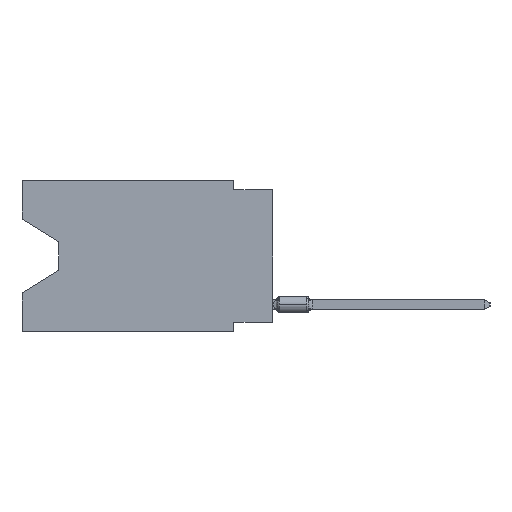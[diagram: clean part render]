
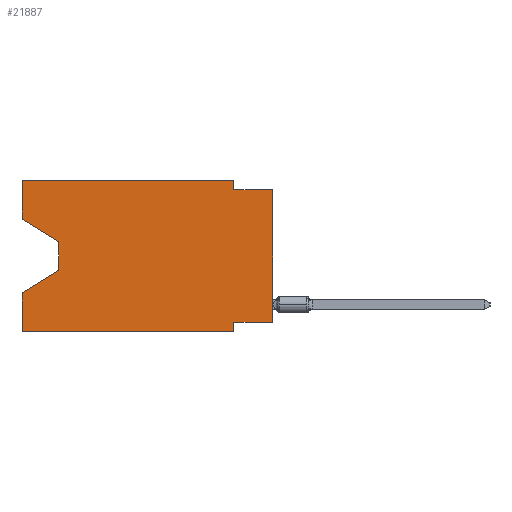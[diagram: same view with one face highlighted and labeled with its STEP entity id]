
A CAD part, left-side view. The second image highlights one B-rep face of the part: STEP entity #21887.
In plain terms, the highlighted planar face has unit normal (-1, 0, 0).
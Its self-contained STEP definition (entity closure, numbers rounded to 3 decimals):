
#831 = VERTEX_POINT ( 'NONE', #34615 ) ;
#1545 = LINE ( 'NONE', #26034, #27329 ) ;
#1785 = CARTESIAN_POINT ( 'NONE',  ( 0., 16.383, -9.906 ) ) ;
#2876 = AXIS2_PLACEMENT_3D ( 'NONE', #51120, #46877, #22471 ) ;
#3183 = LINE ( 'NONE', #36158, #4420 ) ;
#3399 = ORIENTED_EDGE ( 'NONE', *, *, #40823, .T. ) ;
#4256 = ORIENTED_EDGE ( 'NONE', *, *, #48733, .F. ) ;
#4420 = VECTOR ( 'NONE', #36419, 1000. ) ;
#5033 = VERTEX_POINT ( 'NONE', #38835 ) ;
#5280 = CARTESIAN_POINT ( 'NONE',  ( 0., 0., 0. ) ) ;
#5468 = CARTESIAN_POINT ( 'NONE',  ( 0., 0., -9.271 ) ) ;
#7400 = VECTOR ( 'NONE', #24288, 1000. ) ;
#10766 = EDGE_CURVE ( 'NONE', #42158, #831, #1545, .T. ) ;
#10770 = FACE_OUTER_BOUND ( 'NONE', #13644, .T. ) ;
#11017 = ORIENTED_EDGE ( 'NONE', *, *, #44623, .F. ) ;
#11124 = VERTEX_POINT ( 'NONE', #34061 ) ;
#12025 = ORIENTED_EDGE ( 'NONE', *, *, #39941, .T. ) ;
#12533 = CARTESIAN_POINT ( 'NONE',  ( 0., 13.97, -4.013 ) ) ;
#12757 = VERTEX_POINT ( 'NONE', #39662 ) ;
#12951 = VECTOR ( 'NONE', #42785, 1000. ) ;
#13255 = LINE ( 'NONE', #5280, #24822 ) ;
#13481 = ORIENTED_EDGE ( 'NONE', *, *, #10766, .F. ) ;
#13644 = EDGE_LOOP ( 'NONE', ( #12025, #32286, #3399, #4256, #22071, #27933, #26501, #36245, #28026, #23104, #11017, #13481 ) ) ;
#13755 = DIRECTION ( 'NONE',  ( 0., 0., -1. ) ) ;
#15099 = DIRECTION ( 'NONE',  ( 0., 0., 1. ) ) ;
#16007 = VERTEX_POINT ( 'NONE', #45386 ) ;
#16829 = LINE ( 'NONE', #44961, #7400 ) ;
#17113 = VECTOR ( 'NONE', #44923, 1000. ) ;
#17151 = VERTEX_POINT ( 'NONE', #1785 ) ;
#17967 = DIRECTION ( 'NONE',  ( 0., -1., 0. ) ) ;
#19149 = CARTESIAN_POINT ( 'NONE',  ( 0., 2.54, -9.906 ) ) ;
#20970 = VECTOR ( 'NONE', #17967, 1000. ) ;
#21887 = ADVANCED_FACE ( 'NONE', ( #10770 ), #26980, .F. ) ;
#22071 = ORIENTED_EDGE ( 'NONE', *, *, #27393, .T. ) ;
#22471 = DIRECTION ( 'NONE',  ( 0., 0., -1. ) ) ;
#23104 = ORIENTED_EDGE ( 'NONE', *, *, #23711, .F. ) ;
#23711 = EDGE_CURVE ( 'NONE', #16007, #33306, #38208, .T. ) ;
#23868 = LINE ( 'NONE', #39273, #49271 ) ;
#24238 = DIRECTION ( 'NONE',  ( 0., 0.855, -0.519 ) ) ;
#24288 = DIRECTION ( 'NONE',  ( 0., -0.855, -0.519 ) ) ;
#24591 = VECTOR ( 'NONE', #24238, 1000. ) ;
#24822 = VECTOR ( 'NONE', #33198, 1000. ) ;
#25986 = CARTESIAN_POINT ( 'NONE',  ( 0., 16.383, 0. ) ) ;
#26034 = CARTESIAN_POINT ( 'NONE',  ( 0., 16.383, 0. ) ) ;
#26501 = ORIENTED_EDGE ( 'NONE', *, *, #43029, .F. ) ;
#26977 = CARTESIAN_POINT ( 'NONE',  ( 0., 0., -9.271 ) ) ;
#26980 = PLANE ( 'NONE',  #2876 ) ;
#27329 = VECTOR ( 'NONE', #30273, 1000. ) ;
#27393 = EDGE_CURVE ( 'NONE', #17151, #41186, #3183, .T. ) ;
#27529 = EDGE_CURVE ( 'NONE', #36284, #5033, #13255, .T. ) ;
#27933 = ORIENTED_EDGE ( 'NONE', *, *, #32968, .F. ) ;
#27949 = LINE ( 'NONE', #32206, #24591 ) ;
#28026 = ORIENTED_EDGE ( 'NONE', *, *, #46374, .F. ) ;
#28791 = CARTESIAN_POINT ( 'NONE',  ( 0., 16.383, -2.546 ) ) ;
#29689 = DIRECTION ( 'NONE',  ( 0., -1., 0. ) ) ;
#30273 = DIRECTION ( 'NONE',  ( 0., 0., 1. ) ) ;
#31568 = EDGE_CURVE ( 'NONE', #43989, #12757, #32733, .T. ) ;
#31872 = CARTESIAN_POINT ( 'NONE',  ( 0., 13.97, -4.013 ) ) ;
#32206 = CARTESIAN_POINT ( 'NONE',  ( 0., 13.97, -5.893 ) ) ;
#32286 = ORIENTED_EDGE ( 'NONE', *, *, #31568, .T. ) ;
#32733 = LINE ( 'NONE', #12533, #17113 ) ;
#32968 = EDGE_CURVE ( 'NONE', #11124, #41186, #42269, .T. ) ;
#33198 = DIRECTION ( 'NONE',  ( 0., 0., 1. ) ) ;
#33306 = VERTEX_POINT ( 'NONE', #40872 ) ;
#33954 = LINE ( 'NONE', #25986, #50386 ) ;
#34061 = CARTESIAN_POINT ( 'NONE',  ( 0., 2.54, -9.271 ) ) ;
#34615 = CARTESIAN_POINT ( 'NONE',  ( 0., 16.383, 0. ) ) ;
#36158 = CARTESIAN_POINT ( 'NONE',  ( 0., 16.383, -9.906 ) ) ;
#36245 = ORIENTED_EDGE ( 'NONE', *, *, #27529, .T. ) ;
#36284 = VERTEX_POINT ( 'NONE', #26977 ) ;
#36419 = DIRECTION ( 'NONE',  ( 0., -1., 0. ) ) ;
#36614 = VECTOR ( 'NONE', #41606, 1000. ) ;
#38147 = CARTESIAN_POINT ( 'NONE',  ( 0., 0., -0.635 ) ) ;
#38208 = LINE ( 'NONE', #50125, #50786 ) ;
#38287 = CARTESIAN_POINT ( 'NONE',  ( 0., 2.54, -9.906 ) ) ;
#38835 = CARTESIAN_POINT ( 'NONE',  ( 0., 0., -0.635 ) ) ;
#39273 = CARTESIAN_POINT ( 'NONE',  ( 0., 16.383, 0. ) ) ;
#39662 = CARTESIAN_POINT ( 'NONE',  ( 0., 13.97, -5.893 ) ) ;
#39941 = EDGE_CURVE ( 'NONE', #42158, #43989, #16829, .T. ) ;
#40823 = EDGE_CURVE ( 'NONE', #12757, #44434, #27949, .T. ) ;
#40872 = CARTESIAN_POINT ( 'NONE',  ( 0., 2.54, -0.635 ) ) ;
#41186 = VERTEX_POINT ( 'NONE', #19149 ) ;
#41606 = DIRECTION ( 'NONE',  ( 0., 1., 0. ) ) ;
#42158 = VERTEX_POINT ( 'NONE', #28791 ) ;
#42269 = LINE ( 'NONE', #38287, #12951 ) ;
#42785 = DIRECTION ( 'NONE',  ( 0., 0., -1. ) ) ;
#43029 = EDGE_CURVE ( 'NONE', #36284, #11124, #45582, .T. ) ;
#43784 = CARTESIAN_POINT ( 'NONE',  ( 0., 16.383, -7.36 ) ) ;
#43989 = VERTEX_POINT ( 'NONE', #31872 ) ;
#44434 = VERTEX_POINT ( 'NONE', #43784 ) ;
#44623 = EDGE_CURVE ( 'NONE', #831, #16007, #33954, .T. ) ;
#44923 = DIRECTION ( 'NONE',  ( 0., 0., -1. ) ) ;
#44961 = CARTESIAN_POINT ( 'NONE',  ( 0., 16.383, -2.546 ) ) ;
#45386 = CARTESIAN_POINT ( 'NONE',  ( 0., 2.54, 0. ) ) ;
#45582 = LINE ( 'NONE', #5468, #36614 ) ;
#46374 = EDGE_CURVE ( 'NONE', #33306, #5033, #50852, .T. ) ;
#46877 = DIRECTION ( 'NONE',  ( 1., 0., 0. ) ) ;
#48733 = EDGE_CURVE ( 'NONE', #17151, #44434, #23868, .T. ) ;
#49271 = VECTOR ( 'NONE', #15099, 1000. ) ;
#50125 = CARTESIAN_POINT ( 'NONE',  ( 0., 2.54, 0. ) ) ;
#50386 = VECTOR ( 'NONE', #29689, 1000. ) ;
#50786 = VECTOR ( 'NONE', #13755, 1000. ) ;
#50852 = LINE ( 'NONE', #38147, #20970 ) ;
#51120 = CARTESIAN_POINT ( 'NONE',  ( 0., 16.383, 0. ) ) ;
